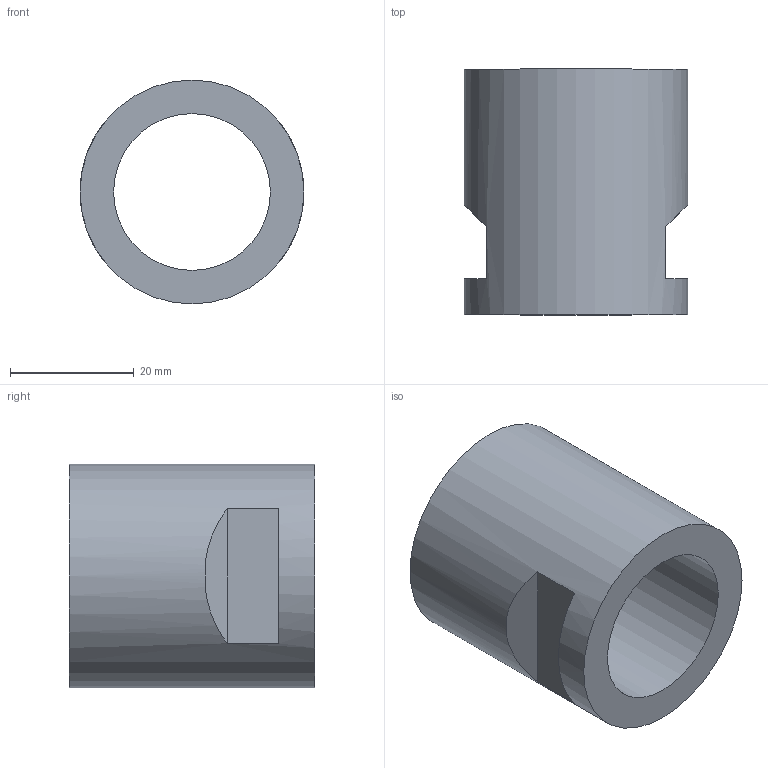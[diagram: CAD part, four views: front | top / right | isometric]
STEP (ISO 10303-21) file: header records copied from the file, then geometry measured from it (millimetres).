
FILE_DESCRIPTION(/* description */ (''),/* implementation_level */ '2;1');
FILE_NAME(/* name */ 'SG22 Barrel Nut Release.step',/* time_stamp */ '2021-03-18T08:53:38-06:00',/* author */ (''),/* organization */ (''),/* preprocessor_version */ 'ST-DEVELOPER v18.1',/* originating_system */ 'Autodesk Translation Framework v9.10.0.1330',/* authorisation */ '');
FILE_SCHEMA (('AUTOMOTIVE_DESIGN { 1 0 10303 214 3 1 1 }'));
Length unit declared in the file: millimetre
Products named in the file (1): Brace V2
Bounding box: 36.25 x 39.78 x 36.25 mm (x, y, z)
Volume: 16281.2 mm3; surface area: 9918.3 mm2
Topology: 1 solids, 1 shells, 81 faces, 211 edges, 134 vertices
Faces by surface type: cone 43, plane 25, cylinder 13
Full cylindrical faces by diameter (mm): 25.391 x1, 30.118 x1, 32.493 x3, 35.56 x1, 36.246 x1
Entity records: 3646 total; most frequent: CARTESIAN_POINT 1753, ORIENTED_EDGE 422, DIRECTION 326, EDGE_CURVE 211, VERTEX_POINT 134, AXIS2_PLACEMENT_3D 121, EDGE_LOOP 85, LINE 84
